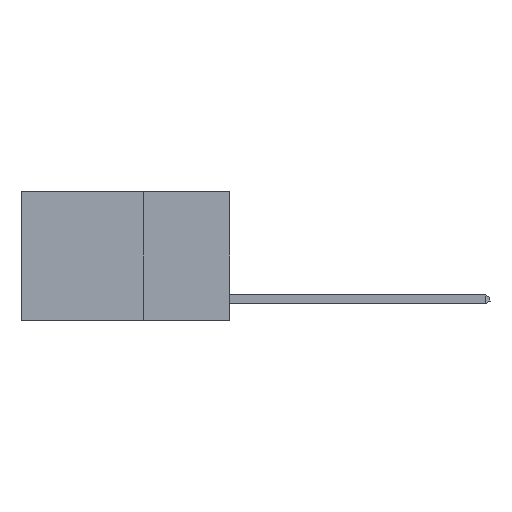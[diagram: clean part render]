
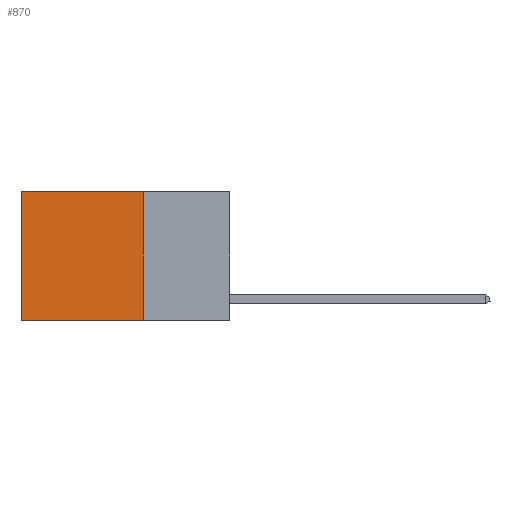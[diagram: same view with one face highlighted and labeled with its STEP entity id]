
A CAD part, left-side view. The second image highlights one B-rep face of the part: STEP entity #870.
In plain terms, the highlighted planar face has unit normal (-1, 0, 0).
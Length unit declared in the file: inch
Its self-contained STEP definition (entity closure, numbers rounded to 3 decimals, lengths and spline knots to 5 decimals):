
#68 = VERTEX_POINT ( 'NONE', #14236 ) ;
#251 = CARTESIAN_POINT ( 'NONE',  ( 0.2625, 0.25, 0. ) ) ;
#733 = CARTESIAN_POINT ( 'NONE',  ( 0.2625, 0.6, -0.37 ) ) ;
#870 = ADVANCED_FACE ( 'NONE', ( #16418 ), #9509, .F. ) ;
#1011 = DIRECTION ( 'NONE',  ( 0., 0., -1. ) ) ;
#1364 = LINE ( 'NONE', #15385, #8602 ) ;
#1819 = DIRECTION ( 'NONE',  ( 1., 0., 0. ) ) ;
#2845 = CARTESIAN_POINT ( 'NONE',  ( 0.2625, 0.25, 0. ) ) ;
#4970 = VERTEX_POINT ( 'NONE', #733 ) ;
#6270 = VERTEX_POINT ( 'NONE', #7250 ) ;
#7130 = CARTESIAN_POINT ( 'NONE',  ( 0.2625, 0.25, -0.37 ) ) ;
#7250 = CARTESIAN_POINT ( 'NONE',  ( 0.2625, 0.25, -0.37 ) ) ;
#8324 = ORIENTED_EDGE ( 'NONE', *, *, #15532, .F. ) ;
#8558 = EDGE_CURVE ( 'NONE', #68, #4970, #12704, .T. ) ;
#8602 = VECTOR ( 'NONE', #16899, 39.37008 ) ;
#8663 = EDGE_CURVE ( 'NONE', #18811, #6270, #18410, .T. ) ;
#9509 = PLANE ( 'NONE',  #15620 ) ;
#9719 = ORIENTED_EDGE ( 'NONE', *, *, #8663, .F. ) ;
#10884 = VECTOR ( 'NONE', #13263, 39.37008 ) ;
#11803 = ORIENTED_EDGE ( 'NONE', *, *, #8558, .T. ) ;
#12642 = DIRECTION ( 'NONE',  ( 0., 0., -1. ) ) ;
#12704 = LINE ( 'NONE', #19472, #17693 ) ;
#13263 = DIRECTION ( 'NONE',  ( 0., 1., 0. ) ) ;
#13636 = DIRECTION ( 'NONE',  ( 0., 0., -1. ) ) ;
#14236 = CARTESIAN_POINT ( 'NONE',  ( 0.2625, 0.6, 0. ) ) ;
#14972 = LINE ( 'NONE', #7130, #10884 ) ;
#15053 = CARTESIAN_POINT ( 'NONE',  ( 0.2625, 0.25, 0. ) ) ;
#15328 = VECTOR ( 'NONE', #13636, 39.37008 ) ;
#15385 = CARTESIAN_POINT ( 'NONE',  ( 0.2625, 0.25, 0. ) ) ;
#15532 = EDGE_CURVE ( 'NONE', #6270, #4970, #14972, .T. ) ;
#15620 = AXIS2_PLACEMENT_3D ( 'NONE', #251, #1819, #12642 ) ;
#16418 = FACE_OUTER_BOUND ( 'NONE', #19896, .T. ) ;
#16899 = DIRECTION ( 'NONE',  ( 0., 1., 0. ) ) ;
#16921 = ORIENTED_EDGE ( 'NONE', *, *, #18265, .T. ) ;
#17693 = VECTOR ( 'NONE', #1011, 39.37008 ) ;
#18265 = EDGE_CURVE ( 'NONE', #18811, #68, #1364, .T. ) ;
#18410 = LINE ( 'NONE', #2845, #15328 ) ;
#18811 = VERTEX_POINT ( 'NONE', #15053 ) ;
#19472 = CARTESIAN_POINT ( 'NONE',  ( 0.2625, 0.6, 0. ) ) ;
#19896 = EDGE_LOOP ( 'NONE', ( #11803, #8324, #9719, #16921 ) ) ;
